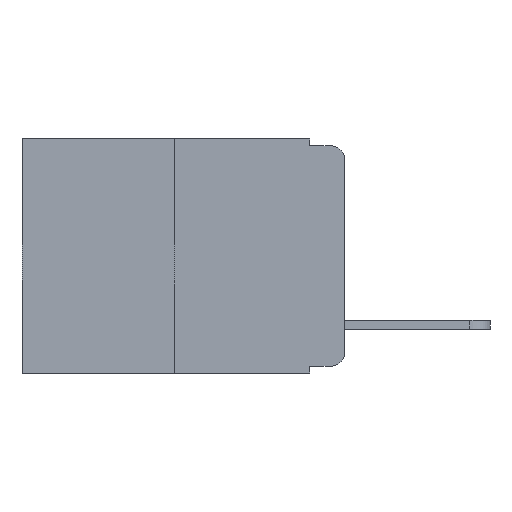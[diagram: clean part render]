
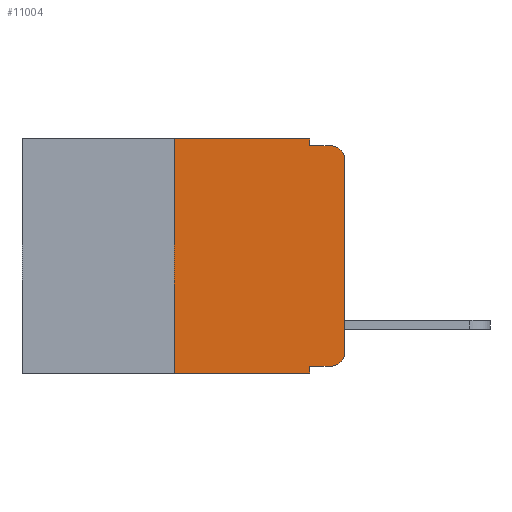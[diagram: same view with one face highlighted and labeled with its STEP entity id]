
A CAD part, left-side view. The second image highlights one B-rep face of the part: STEP entity #11004.
In plain terms, the highlighted planar face has unit normal (-1, 0, 0).
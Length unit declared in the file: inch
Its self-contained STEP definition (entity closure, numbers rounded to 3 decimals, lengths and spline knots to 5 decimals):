
#132 = VERTEX_POINT ( 'NONE', #5357 ) ;
#583 = DIRECTION ( 'NONE',  ( -1., 0., 0. ) ) ;
#693 = EDGE_CURVE ( 'NONE', #7242, #2850, #5933, .T. ) ;
#805 = LINE ( 'NONE', #14403, #13323 ) ;
#1086 = EDGE_CURVE ( 'NONE', #11654, #6139, #6650, .T. ) ;
#1114 = EDGE_CURVE ( 'NONE', #10307, #3292, #9407, .T. ) ;
#1374 = DIRECTION ( 'NONE',  ( 0., 0., 1. ) ) ;
#1539 = AXIS2_PLACEMENT_3D ( 'NONE', #5116, #13370, #6296 ) ;
#1767 = CARTESIAN_POINT ( 'NONE',  ( 0., 0.473, 0. ) ) ;
#2435 = VECTOR ( 'NONE', #6533, 39.37008 ) ;
#2493 = CARTESIAN_POINT ( 'NONE',  ( 0., 0.25, -0.343 ) ) ;
#2850 = VERTEX_POINT ( 'NONE', #4926 ) ;
#2879 = ORIENTED_EDGE ( 'NONE', *, *, #12230, .F. ) ;
#2968 = EDGE_CURVE ( 'NONE', #10307, #11654, #805, .T. ) ;
#3011 = ORIENTED_EDGE ( 'NONE', *, *, #2968, .F. ) ;
#3292 = VERTEX_POINT ( 'NONE', #7138 ) ;
#3903 = VECTOR ( 'NONE', #12214, 39.37008 ) ;
#3955 = DIRECTION ( 'NONE',  ( 0., -1., 0. ) ) ;
#4021 = CIRCLE ( 'NONE', #8077, 0.02 ) ;
#4179 = CARTESIAN_POINT ( 'NONE',  ( 0., 0.051, 0. ) ) ;
#4295 = EDGE_CURVE ( 'NONE', #7276, #3292, #13122, .T. ) ;
#4926 = CARTESIAN_POINT ( 'NONE',  ( 0., 0.02, -0.01 ) ) ;
#5116 = CARTESIAN_POINT ( 'NONE',  ( 0., 0.02, -0.313 ) ) ;
#5357 = CARTESIAN_POINT ( 'NONE',  ( 0., 0.02, -0.333 ) ) ;
#5658 = VECTOR ( 'NONE', #1374, 39.37008 ) ;
#5780 = ORIENTED_EDGE ( 'NONE', *, *, #6728, .T. ) ;
#5854 = DIRECTION ( 'NONE',  ( 0., -1., 0. ) ) ;
#5933 = LINE ( 'NONE', #9242, #14924 ) ;
#6009 = DIRECTION ( 'NONE',  ( 1., 0., 0. ) ) ;
#6139 = VERTEX_POINT ( 'NONE', #10243 ) ;
#6296 = DIRECTION ( 'NONE',  ( 0., 0., -1. ) ) ;
#6500 = CIRCLE ( 'NONE', #1539, 0.02 ) ;
#6533 = DIRECTION ( 'NONE',  ( 0., 0., -1. ) ) ;
#6568 = EDGE_CURVE ( 'NONE', #10822, #2850, #4021, .T. ) ;
#6650 = LINE ( 'NONE', #1767, #13304 ) ;
#6728 = EDGE_CURVE ( 'NONE', #7276, #132, #14301, .T. ) ;
#6839 = AXIS2_PLACEMENT_3D ( 'NONE', #10725, #6009, #14243 ) ;
#6846 = CARTESIAN_POINT ( 'NONE',  ( 0., 0., -0.03 ) ) ;
#7138 = CARTESIAN_POINT ( 'NONE',  ( 0., 0.051, -0.343 ) ) ;
#7242 = VERTEX_POINT ( 'NONE', #11145 ) ;
#7276 = VERTEX_POINT ( 'NONE', #14718 ) ;
#7604 = CARTESIAN_POINT ( 'NONE',  ( 0., 0.02, -0.03 ) ) ;
#7778 = ORIENTED_EDGE ( 'NONE', *, *, #1114, .T. ) ;
#7903 = DIRECTION ( 'NONE',  ( 0., -1., 0. ) ) ;
#8066 = CARTESIAN_POINT ( 'NONE',  ( 0., 0.473, -0.343 ) ) ;
#8077 = AXIS2_PLACEMENT_3D ( 'NONE', #7604, #583, #8790 ) ;
#8228 = EDGE_LOOP ( 'NONE', ( #13429, #11823, #8881, #2879, #10402, #3011, #7778, #14950, #5780, #8380 ) ) ;
#8380 = ORIENTED_EDGE ( 'NONE', *, *, #11483, .T. ) ;
#8630 = EDGE_CURVE ( 'NONE', #9062, #10822, #8807, .T. ) ;
#8790 = DIRECTION ( 'NONE',  ( 0., 0., -1. ) ) ;
#8807 = LINE ( 'NONE', #10683, #5658 ) ;
#8881 = ORIENTED_EDGE ( 'NONE', *, *, #693, .F. ) ;
#9062 = VERTEX_POINT ( 'NONE', #12785 ) ;
#9242 = CARTESIAN_POINT ( 'NONE',  ( 0., 0.051, -0.01 ) ) ;
#9407 = LINE ( 'NONE', #8066, #3903 ) ;
#9980 = VECTOR ( 'NONE', #10750, 39.37008 ) ;
#10243 = CARTESIAN_POINT ( 'NONE',  ( 0., 0.051, 0. ) ) ;
#10307 = VERTEX_POINT ( 'NONE', #2493 ) ;
#10378 = FACE_OUTER_BOUND ( 'NONE', #8228, .T. ) ;
#10402 = ORIENTED_EDGE ( 'NONE', *, *, #1086, .F. ) ;
#10683 = CARTESIAN_POINT ( 'NONE',  ( 0., 0., 0. ) ) ;
#10725 = CARTESIAN_POINT ( 'NONE',  ( 0., 0.473, 0. ) ) ;
#10750 = DIRECTION ( 'NONE',  ( 0., 0., -1. ) ) ;
#10784 = CARTESIAN_POINT ( 'NONE',  ( 0., 0.051, 0. ) ) ;
#10822 = VERTEX_POINT ( 'NONE', #6846 ) ;
#11004 = ADVANCED_FACE ( 'NONE', ( #10378 ), #13089, .F. ) ;
#11145 = CARTESIAN_POINT ( 'NONE',  ( 0., 0.051, -0.01 ) ) ;
#11432 = CARTESIAN_POINT ( 'NONE',  ( 0., 0.051, -0.333 ) ) ;
#11483 = EDGE_CURVE ( 'NONE', #132, #9062, #6500, .T. ) ;
#11654 = VERTEX_POINT ( 'NONE', #12498 ) ;
#11823 = ORIENTED_EDGE ( 'NONE', *, *, #6568, .T. ) ;
#11832 = LINE ( 'NONE', #4179, #2435 ) ;
#12214 = DIRECTION ( 'NONE',  ( 0., -1., 0. ) ) ;
#12230 = EDGE_CURVE ( 'NONE', #6139, #7242, #11832, .T. ) ;
#12498 = CARTESIAN_POINT ( 'NONE',  ( 0., 0.25, 0. ) ) ;
#12785 = CARTESIAN_POINT ( 'NONE',  ( 0., 0., -0.313 ) ) ;
#13089 = PLANE ( 'NONE',  #6839 ) ;
#13122 = LINE ( 'NONE', #10784, #9980 ) ;
#13304 = VECTOR ( 'NONE', #3955, 39.37008 ) ;
#13323 = VECTOR ( 'NONE', #14477, 39.37008 ) ;
#13370 = DIRECTION ( 'NONE',  ( -1., 0., 0. ) ) ;
#13429 = ORIENTED_EDGE ( 'NONE', *, *, #8630, .T. ) ;
#13945 = VECTOR ( 'NONE', #7903, 39.37008 ) ;
#14243 = DIRECTION ( 'NONE',  ( 0., 0., -1. ) ) ;
#14301 = LINE ( 'NONE', #11432, #13945 ) ;
#14403 = CARTESIAN_POINT ( 'NONE',  ( 0., 0.25, 0. ) ) ;
#14477 = DIRECTION ( 'NONE',  ( 0., 0., 1. ) ) ;
#14718 = CARTESIAN_POINT ( 'NONE',  ( 0., 0.051, -0.333 ) ) ;
#14924 = VECTOR ( 'NONE', #5854, 39.37008 ) ;
#14950 = ORIENTED_EDGE ( 'NONE', *, *, #4295, .F. ) ;
